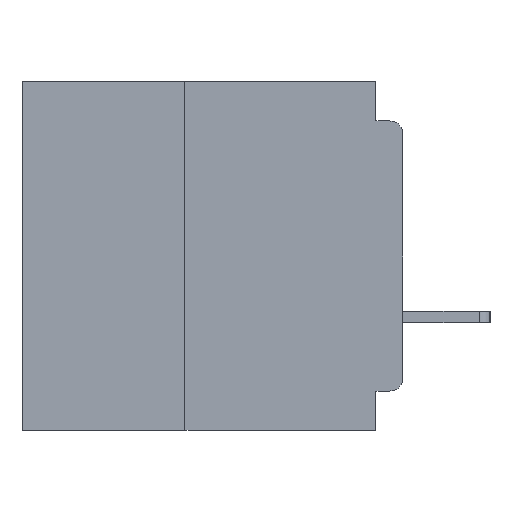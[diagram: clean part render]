
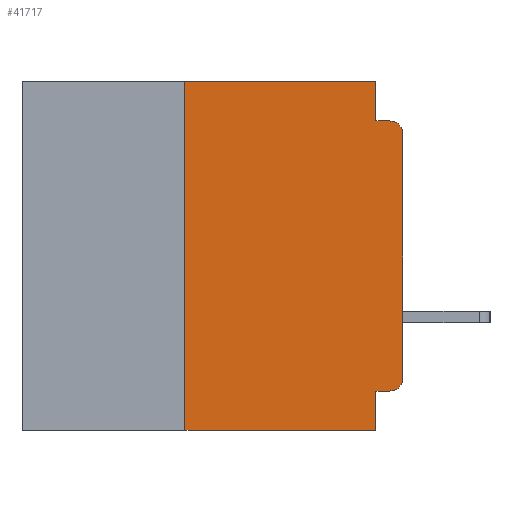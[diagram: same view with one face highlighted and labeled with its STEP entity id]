
A CAD part, left-side view. The second image highlights one B-rep face of the part: STEP entity #41717.
In plain terms, the highlighted planar face has unit normal (-1, 0, 0).
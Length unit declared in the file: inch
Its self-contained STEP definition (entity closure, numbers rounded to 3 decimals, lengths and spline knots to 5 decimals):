
#738 = VECTOR ( 'NONE', #52188, 39.37008 ) ;
#1048 = DIRECTION ( 'NONE',  ( -1., 0., 0. ) ) ;
#1295 = VERTEX_POINT ( 'NONE', #44981 ) ;
#3617 = ORIENTED_EDGE ( 'NONE', *, *, #54433, .F. ) ;
#3651 = CARTESIAN_POINT ( 'NONE',  ( 0., 0., -0.34 ) ) ;
#3836 = EDGE_CURVE ( 'NONE', #25285, #11203, #37489, .T. ) ;
#4070 = CARTESIAN_POINT ( 'NONE',  ( 0., 0.031, -0.355 ) ) ;
#4285 = CARTESIAN_POINT ( 'NONE',  ( 0., 0.015, -0.045 ) ) ;
#4292 = ORIENTED_EDGE ( 'NONE', *, *, #54088, .T. ) ;
#4873 = VERTEX_POINT ( 'NONE', #29612 ) ;
#5027 = ORIENTED_EDGE ( 'NONE', *, *, #50166, .F. ) ;
#5807 = DIRECTION ( 'NONE',  ( 0., 0., 1. ) ) ;
#9278 = ORIENTED_EDGE ( 'NONE', *, *, #3836, .T. ) ;
#9917 = CARTESIAN_POINT ( 'NONE',  ( 0., 0.031, 0. ) ) ;
#11203 = VERTEX_POINT ( 'NONE', #20317 ) ;
#11691 = DIRECTION ( 'NONE',  ( 0., 0., -1. ) ) ;
#12428 = DIRECTION ( 'NONE',  ( 0., 1., 0. ) ) ;
#12664 = VERTEX_POINT ( 'NONE', #4285 ) ;
#12801 = CARTESIAN_POINT ( 'NONE',  ( 0., 0.437, 0. ) ) ;
#13015 = CARTESIAN_POINT ( 'NONE',  ( 0., 0.015, -0.34 ) ) ;
#13319 = DIRECTION ( 'NONE',  ( 0., -1., 0. ) ) ;
#13600 = VECTOR ( 'NONE', #34838, 39.37008 ) ;
#16566 = VECTOR ( 'NONE', #5807, 39.37008 ) ;
#17059 = VECTOR ( 'NONE', #12428, 39.37008 ) ;
#17574 = DIRECTION ( 'NONE',  ( 0., 0., -1. ) ) ;
#17827 = VECTOR ( 'NONE', #24221, 39.37008 ) ;
#19695 = CARTESIAN_POINT ( 'NONE',  ( 0., 0.031, 0. ) ) ;
#20317 = CARTESIAN_POINT ( 'NONE',  ( 0., 0.031, -0.4 ) ) ;
#22652 = DIRECTION ( 'NONE',  ( 0., -1., 0. ) ) ;
#23196 = CARTESIAN_POINT ( 'NONE',  ( 0., 0.25, -0.4 ) ) ;
#24221 = DIRECTION ( 'NONE',  ( 0., 0., -1. ) ) ;
#24236 = VECTOR ( 'NONE', #13319, 39.37008 ) ;
#24851 = LINE ( 'NONE', #30067, #738 ) ;
#25285 = VERTEX_POINT ( 'NONE', #23196 ) ;
#25515 = VERTEX_POINT ( 'NONE', #42637 ) ;
#26274 = EDGE_CURVE ( 'NONE', #4873, #46253, #42224, .T. ) ;
#26752 = CARTESIAN_POINT ( 'NONE',  ( 0., 0.437, -0.4 ) ) ;
#26972 = ORIENTED_EDGE ( 'NONE', *, *, #47572, .T. ) ;
#27685 = ORIENTED_EDGE ( 'NONE', *, *, #29815, .F. ) ;
#28144 = CARTESIAN_POINT ( 'NONE',  ( 0., 0.015, -0.06 ) ) ;
#28411 = AXIS2_PLACEMENT_3D ( 'NONE', #28144, #1048, #32635 ) ;
#28561 = LINE ( 'NONE', #50150, #16566 ) ;
#28757 = AXIS2_PLACEMENT_3D ( 'NONE', #13015, #44277, #17574 ) ;
#29612 = CARTESIAN_POINT ( 'NONE',  ( 0., 0.015, -0.355 ) ) ;
#29634 = CARTESIAN_POINT ( 'NONE',  ( 0., 0.437, 0. ) ) ;
#29738 = CARTESIAN_POINT ( 'NONE',  ( 0., 0., -0.06 ) ) ;
#29815 = EDGE_CURVE ( 'NONE', #25515, #39481, #30345, .T. ) ;
#30067 = CARTESIAN_POINT ( 'NONE',  ( 0., 0.031, -0.4 ) ) ;
#30345 = LINE ( 'NONE', #12801, #52365 ) ;
#30363 = CARTESIAN_POINT ( 'NONE',  ( 0., 0., 0. ) ) ;
#32564 = ORIENTED_EDGE ( 'NONE', *, *, #38312, .F. ) ;
#32635 = DIRECTION ( 'NONE',  ( 0., 0., -1. ) ) ;
#34130 = PLANE ( 'NONE',  #34902 ) ;
#34838 = DIRECTION ( 'NONE',  ( 0., 0., 1. ) ) ;
#34902 = AXIS2_PLACEMENT_3D ( 'NONE', #29634, #38557, #11691 ) ;
#35034 = EDGE_CURVE ( 'NONE', #46253, #11203, #24851, .T. ) ;
#35417 = DIRECTION ( 'NONE',  ( 0., -1., 0. ) ) ;
#35751 = CIRCLE ( 'NONE', #28411, 0.015 ) ;
#37489 = LINE ( 'NONE', #26752, #24236 ) ;
#38312 = EDGE_CURVE ( 'NONE', #1295, #12664, #48339, .T. ) ;
#38557 = DIRECTION ( 'NONE',  ( 1., 0., 0. ) ) ;
#39481 = VERTEX_POINT ( 'NONE', #9917 ) ;
#40153 = ORIENTED_EDGE ( 'NONE', *, *, #48379, .T. ) ;
#41717 = ADVANCED_FACE ( 'NONE', ( #42858 ), #34130, .F. ) ;
#42224 = LINE ( 'NONE', #56892, #17059 ) ;
#42637 = CARTESIAN_POINT ( 'NONE',  ( 0., 0.25, 0. ) ) ;
#42858 = FACE_OUTER_BOUND ( 'NONE', #44553, .T. ) ;
#44277 = DIRECTION ( 'NONE',  ( -1., 0., 0. ) ) ;
#44553 = EDGE_LOOP ( 'NONE', ( #4292, #40153, #32564, #3617, #27685, #5027, #9278, #44985, #49107, #26972 ) ) ;
#44789 = CARTESIAN_POINT ( 'NONE',  ( 0., 0., -0.045 ) ) ;
#44890 = VERTEX_POINT ( 'NONE', #29738 ) ;
#44981 = CARTESIAN_POINT ( 'NONE',  ( 0., 0.031, -0.045 ) ) ;
#44985 = ORIENTED_EDGE ( 'NONE', *, *, #35034, .F. ) ;
#46253 = VERTEX_POINT ( 'NONE', #4070 ) ;
#47572 = EDGE_CURVE ( 'NONE', #4873, #48182, #56445, .T. ) ;
#48182 = VERTEX_POINT ( 'NONE', #3651 ) ;
#48339 = LINE ( 'NONE', #44789, #57206 ) ;
#48379 = EDGE_CURVE ( 'NONE', #44890, #12664, #35751, .T. ) ;
#49107 = ORIENTED_EDGE ( 'NONE', *, *, #26274, .F. ) ;
#49165 = LINE ( 'NONE', #30363, #13600 ) ;
#50150 = CARTESIAN_POINT ( 'NONE',  ( 0., 0.25, -0.4 ) ) ;
#50166 = EDGE_CURVE ( 'NONE', #25285, #25515, #28561, .T. ) ;
#52188 = DIRECTION ( 'NONE',  ( 0., 0., -1. ) ) ;
#52365 = VECTOR ( 'NONE', #35417, 39.37008 ) ;
#54088 = EDGE_CURVE ( 'NONE', #48182, #44890, #49165, .T. ) ;
#54433 = EDGE_CURVE ( 'NONE', #39481, #1295, #55994, .T. ) ;
#55994 = LINE ( 'NONE', #19695, #17827 ) ;
#56445 = CIRCLE ( 'NONE', #28757, 0.015 ) ;
#56892 = CARTESIAN_POINT ( 'NONE',  ( 0., 0., -0.355 ) ) ;
#57206 = VECTOR ( 'NONE', #22652, 39.37008 ) ;
